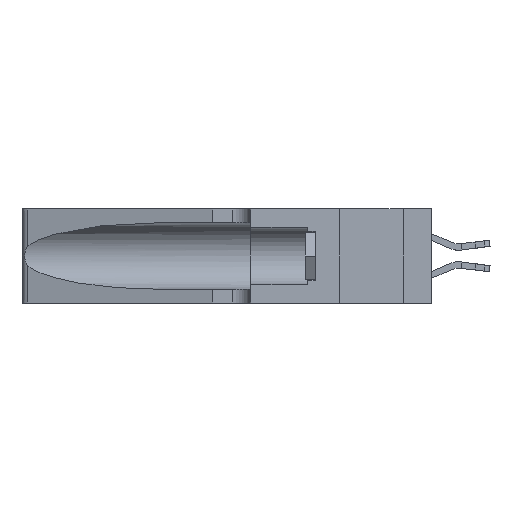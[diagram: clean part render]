
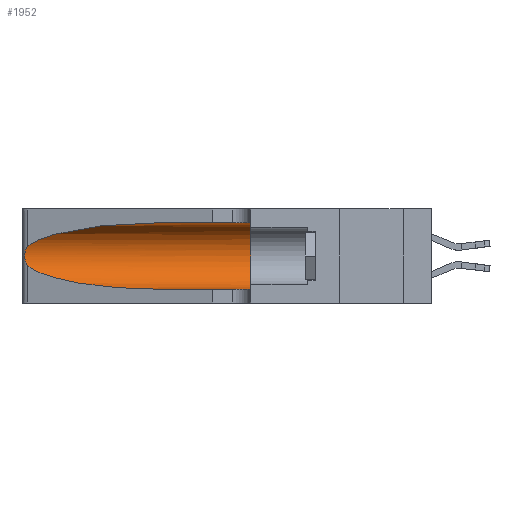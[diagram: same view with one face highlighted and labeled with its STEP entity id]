
A CAD part, left-side view. The second image highlights one B-rep face of the part: STEP entity #1952.
In plain terms, the highlighted cylindrical face has radius 3.308 mm (diameter 6.617 mm), a partial arc.
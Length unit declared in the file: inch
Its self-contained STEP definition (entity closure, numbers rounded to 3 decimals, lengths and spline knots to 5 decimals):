
#855 = CARTESIAN_POINT ( 'NONE',  ( 0.1305, 0.72297, 0.05475 ) ) ;
#1093 = CARTESIAN_POINT ( 'NONE',  ( 0.1305, 0.35, 0.185 ) ) ;
#1400 = EDGE_CURVE ( 'NONE', #22388, #14040, #3299, .T. ) ;
#1952 = ADVANCED_FACE ( 'NONE', ( #19445 ), #23767, .F. ) ;
#2229 = DIRECTION ( 'NONE',  ( 0., -1., 0. ) ) ;
#2430 = ORIENTED_EDGE ( 'NONE', *, *, #17241, .F. ) ;
#3299 = B_SPLINE_CURVE_WITH_KNOTS ( 'NONE', 3,
 ( #21216, #11047, #3499, #6038, #26441, #29686, #29442, #26988, #22116, #3950, #3842, #14441, #16661, #9284 ),
 .UNSPECIFIED., .F., .F.,
 ( 4, 2, 2, 2, 2, 2, 4 ),
 ( 0., 0.00027, 0.00053, 0.00107, 0.0016, 0.00187, 0.00214 ),
 .UNSPECIFIED. ) ;
#3499 = CARTESIAN_POINT ( 'NONE',  ( 0.25639, 1.23184, 0.21858 ) ) ;
#3841 = ORIENTED_EDGE ( 'NONE', *, *, #13511, .T. ) ;
#3842 = CARTESIAN_POINT ( 'NONE',  ( 0.25789, 1.23486, 0.15765 ) ) ;
#3950 = CARTESIAN_POINT ( 'NONE',  ( 0.25856, 1.23593, 0.16098 ) ) ;
#4082 = DIRECTION ( 'NONE',  ( 0., 1., 0. ) ) ;
#4876 = CARTESIAN_POINT ( 'NONE',  ( 0.1305, 0.35, 0.31525 ) ) ;
#5191 = CARTESIAN_POINT ( 'NONE',  ( 0.2373, 1.15595, 0.08982 ) ) ;
#6038 = CARTESIAN_POINT ( 'NONE',  ( 0.25787, 1.23484, 0.2124 ) ) ;
#6069 = LINE ( 'NONE', #10521, #7667 ) ;
#6358 = VECTOR ( 'NONE', #2229, 39.37008 ) ;
#7667 = VECTOR ( 'NONE', #13289, 39.37008 ) ;
#9106 = CARTESIAN_POINT ( 'NONE',  ( 0.1305, 1.61858, 0.185 ) ) ;
#9284 = CARTESIAN_POINT ( 'NONE',  ( 0.25487, 1.22718, 0.14631 ) ) ;
#9961 = LINE ( 'NONE', #27134, #6358 ) ;
#10298 = ORIENTED_EDGE ( 'NONE', *, *, #1400, .T. ) ;
#10521 = CARTESIAN_POINT ( 'NONE',  ( 0.1305, 1.61858, 0.05475 ) ) ;
#10805 = AXIS2_PLACEMENT_3D ( 'NONE', #1093, #4082, #31937 ) ;
#10869 = EDGE_CURVE ( 'NONE', #14040, #24514, #17057, .T. ) ;
#10964 = EDGE_LOOP ( 'NONE', ( #26932, #10298, #11010, #3841, #18790, #2430 ) ) ;
#11010 = ORIENTED_EDGE ( 'NONE', *, *, #10869, .T. ) ;
#11047 = CARTESIAN_POINT ( 'NONE',  ( 0.25555, 1.22994, 0.2215 ) ) ;
#11682 = DIRECTION ( 'NONE',  ( 0., -1., 0. ) ) ;
#12713 = CARTESIAN_POINT ( 'NONE',  ( 0.1305, 0.72297, 0.05475 ) ) ;
#13289 = DIRECTION ( 'NONE',  ( 0., -1., 0. ) ) ;
#13511 = EDGE_CURVE ( 'NONE', #24514, #21435, #6069, .T. ) ;
#14040 = VERTEX_POINT ( 'NONE', #27559 ) ;
#14441 = CARTESIAN_POINT ( 'NONE',  ( 0.25639, 1.23186, 0.15144 ) ) ;
#14959 = CARTESIAN_POINT ( 'NONE',  ( 0.18966, 0.96281, 0.31525 ) ) ;
#15277 = CARTESIAN_POINT ( 'NONE',  ( 0.25487, 1.22718, 0.22369 ) ) ;
#15768 =( BOUNDED_CURVE ( )  B_SPLINE_CURVE ( 3, ( #22552, #14959, #18280, #15277 ),
 .UNSPECIFIED., .F., .F. ) 
 B_SPLINE_CURVE_WITH_KNOTS ( ( 4, 4 ),
 ( 1.5708, 2.84003 ),
 .UNSPECIFIED. ) 
 CURVE ( )  GEOMETRIC_REPRESENTATION_ITEM ( )  RATIONAL_B_SPLINE_CURVE ( ( 1., 0.87, 0.87, 1. ) ) 
 REPRESENTATION_ITEM ( '' )  );
#16616 = AXIS2_PLACEMENT_3D ( 'NONE', #9106, #11682, #29503 ) ;
#16661 = CARTESIAN_POINT ( 'NONE',  ( 0.25555, 1.22993, 0.14849 ) ) ;
#17057 =( BOUNDED_CURVE ( )  B_SPLINE_CURVE ( 3, ( #30063, #5191, #28124, #855 ),
 .UNSPECIFIED., .F., .T. ) 
 B_SPLINE_CURVE_WITH_KNOTS ( ( 4, 4 ),
 ( 3.44316, 4.71239 ),
 .UNSPECIFIED. ) 
 CURVE ( )  GEOMETRIC_REPRESENTATION_ITEM ( )  RATIONAL_B_SPLINE_CURVE ( ( 1., 0.87, 0.87, 1. ) ) 
 REPRESENTATION_ITEM ( '' )  );
#17241 = EDGE_CURVE ( 'NONE', #19527, #29130, #9961, .T. ) ;
#18280 = CARTESIAN_POINT ( 'NONE',  ( 0.2373, 1.15595, 0.28018 ) ) ;
#18790 = ORIENTED_EDGE ( 'NONE', *, *, #19649, .F. ) ;
#19445 = FACE_OUTER_BOUND ( 'NONE', #10964, .T. ) ;
#19527 = VERTEX_POINT ( 'NONE', #19852 ) ;
#19649 = EDGE_CURVE ( 'NONE', #29130, #21435, #21385, .T. ) ;
#19852 = CARTESIAN_POINT ( 'NONE',  ( 0.1305, 0.72297, 0.31525 ) ) ;
#21216 = CARTESIAN_POINT ( 'NONE',  ( 0.25487, 1.22718, 0.22369 ) ) ;
#21385 = CIRCLE ( 'NONE', #10805, 0.13025 ) ;
#21435 = VERTEX_POINT ( 'NONE', #31049 ) ;
#22116 = CARTESIAN_POINT ( 'NONE',  ( 0.26017, 1.23833, 0.17102 ) ) ;
#22388 = VERTEX_POINT ( 'NONE', #22465 ) ;
#22465 = CARTESIAN_POINT ( 'NONE',  ( 0.25487, 1.22718, 0.22369 ) ) ;
#22552 = CARTESIAN_POINT ( 'NONE',  ( 0.1305, 0.72297, 0.31525 ) ) ;
#23767 = CYLINDRICAL_SURFACE ( 'NONE', #16616, 0.13025 ) ;
#24514 = VERTEX_POINT ( 'NONE', #12713 ) ;
#26441 = CARTESIAN_POINT ( 'NONE',  ( 0.25854, 1.2359, 0.20912 ) ) ;
#26726 = EDGE_CURVE ( 'NONE', #19527, #22388, #15768, .T. ) ;
#26932 = ORIENTED_EDGE ( 'NONE', *, *, #26726, .T. ) ;
#26988 = CARTESIAN_POINT ( 'NONE',  ( 0.26075, 1.23896, 0.178 ) ) ;
#27134 = CARTESIAN_POINT ( 'NONE',  ( 0.1305, 1.61858, 0.31525 ) ) ;
#27559 = CARTESIAN_POINT ( 'NONE',  ( 0.25487, 1.22718, 0.14631 ) ) ;
#28124 = CARTESIAN_POINT ( 'NONE',  ( 0.18966, 0.96281, 0.05475 ) ) ;
#29130 = VERTEX_POINT ( 'NONE', #4876 ) ;
#29442 = CARTESIAN_POINT ( 'NONE',  ( 0.26075, 1.23896, 0.19203 ) ) ;
#29503 = DIRECTION ( 'NONE',  ( 0., 0., -1. ) ) ;
#29686 = CARTESIAN_POINT ( 'NONE',  ( 0.26018, 1.23835, 0.19895 ) ) ;
#30063 = CARTESIAN_POINT ( 'NONE',  ( 0.25487, 1.22718, 0.14631 ) ) ;
#31049 = CARTESIAN_POINT ( 'NONE',  ( 0.1305, 0.35, 0.05475 ) ) ;
#31937 = DIRECTION ( 'NONE',  ( 0., 0., 1. ) ) ;
